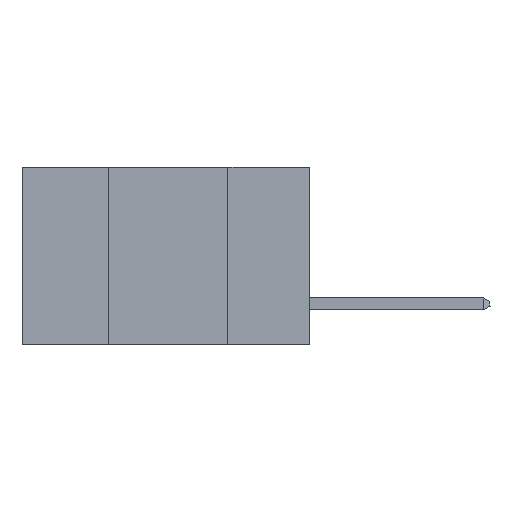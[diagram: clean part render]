
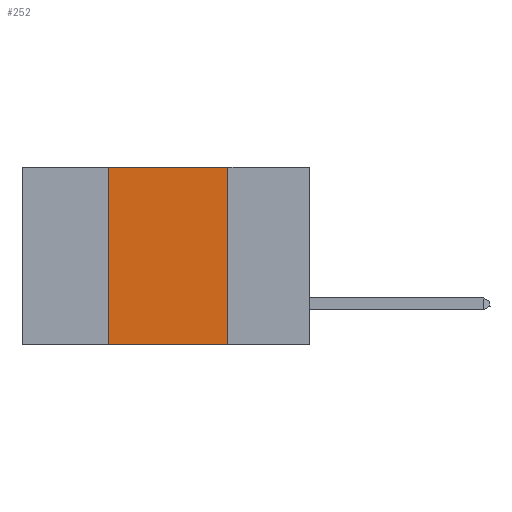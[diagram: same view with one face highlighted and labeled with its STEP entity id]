
A CAD part, left-side view. The second image highlights one B-rep face of the part: STEP entity #252.
In plain terms, the highlighted planar face has unit normal (-1, 0, 0).
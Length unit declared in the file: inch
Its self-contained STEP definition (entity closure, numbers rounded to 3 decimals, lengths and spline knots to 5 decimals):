
#252 = ADVANCED_FACE ( 'NONE', ( #27527 ), #4494, .F. ) ;
#263 = LINE ( 'NONE', #7552, #16024 ) ;
#774 = CARTESIAN_POINT ( 'NONE',  ( 0., 0.17, -0.37 ) ) ;
#1508 = EDGE_CURVE ( 'NONE', #23334, #21971, #263, .T. ) ;
#4074 = EDGE_CURVE ( 'NONE', #23334, #4585, #15867, .T. ) ;
#4106 = EDGE_CURVE ( 'NONE', #4585, #22565, #34019, .T. ) ;
#4339 = ORIENTED_EDGE ( 'NONE', *, *, #1508, .T. ) ;
#4494 = PLANE ( 'NONE',  #27440 ) ;
#4585 = VERTEX_POINT ( 'NONE', #17815 ) ;
#7277 = EDGE_LOOP ( 'NONE', ( #13115, #16912, #7657, #4339 ) ) ;
#7552 = CARTESIAN_POINT ( 'NONE',  ( 0., 0.6, -0.37 ) ) ;
#7657 = ORIENTED_EDGE ( 'NONE', *, *, #4074, .F. ) ;
#7719 = CARTESIAN_POINT ( 'NONE',  ( 0., 0.42, 0. ) ) ;
#9702 = CARTESIAN_POINT ( 'NONE',  ( 0., 0.6, 0. ) ) ;
#9755 = VECTOR ( 'NONE', #23277, 39.37008 ) ;
#12281 = DIRECTION ( 'NONE',  ( 0., 0., -1. ) ) ;
#13115 = ORIENTED_EDGE ( 'NONE', *, *, #28397, .F. ) ;
#14335 = LINE ( 'NONE', #33992, #9755 ) ;
#15281 = DIRECTION ( 'NONE',  ( 0., 0., 1. ) ) ;
#15867 = LINE ( 'NONE', #7719, #19163 ) ;
#16024 = VECTOR ( 'NONE', #28208, 39.37008 ) ;
#16912 = ORIENTED_EDGE ( 'NONE', *, *, #4106, .F. ) ;
#17815 = CARTESIAN_POINT ( 'NONE',  ( 0., 0.42, 0. ) ) ;
#19163 = VECTOR ( 'NONE', #15281, 39.37008 ) ;
#21330 = CARTESIAN_POINT ( 'NONE',  ( 0., 0.17, 0. ) ) ;
#21971 = VERTEX_POINT ( 'NONE', #774 ) ;
#22511 = CARTESIAN_POINT ( 'NONE',  ( 0., 0.42, -0.37 ) ) ;
#22565 = VERTEX_POINT ( 'NONE', #21330 ) ;
#23277 = DIRECTION ( 'NONE',  ( 0., 0., -1. ) ) ;
#23334 = VERTEX_POINT ( 'NONE', #22511 ) ;
#23697 = VECTOR ( 'NONE', #26171, 39.37008 ) ;
#26171 = DIRECTION ( 'NONE',  ( 0., -1., 0. ) ) ;
#27440 = AXIS2_PLACEMENT_3D ( 'NONE', #9702, #28042, #12281 ) ;
#27527 = FACE_OUTER_BOUND ( 'NONE', #7277, .T. ) ;
#28042 = DIRECTION ( 'NONE',  ( 1., 0., 0. ) ) ;
#28208 = DIRECTION ( 'NONE',  ( 0., -1., 0. ) ) ;
#28397 = EDGE_CURVE ( 'NONE', #22565, #21971, #14335, .T. ) ;
#33992 = CARTESIAN_POINT ( 'NONE',  ( 0., 0.17, 0. ) ) ;
#34019 = LINE ( 'NONE', #34040, #23697 ) ;
#34040 = CARTESIAN_POINT ( 'NONE',  ( 0., 0.6, 0. ) ) ;
